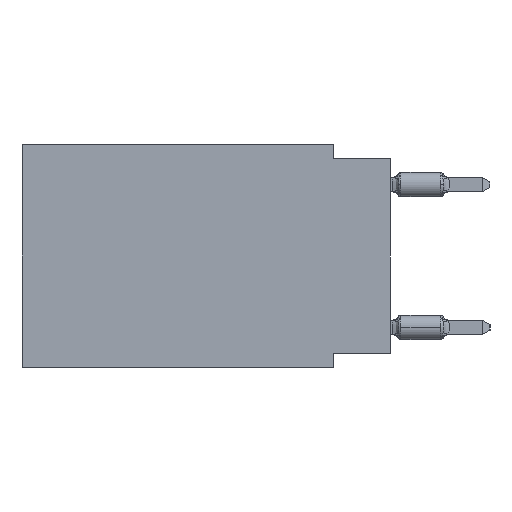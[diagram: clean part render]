
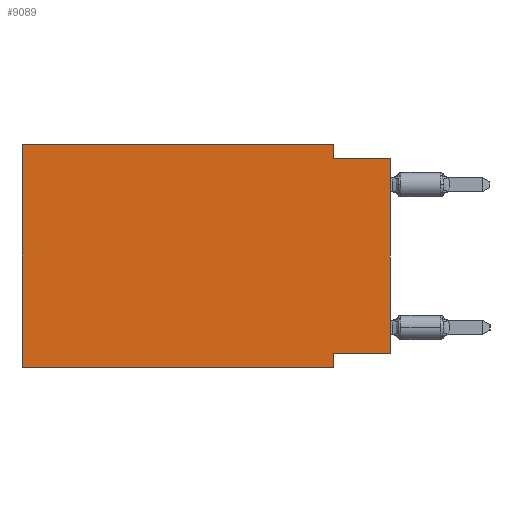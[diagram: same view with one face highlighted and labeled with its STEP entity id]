
A CAD part, left-side view. The second image highlights one B-rep face of the part: STEP entity #9089.
In plain terms, the highlighted planar face has unit normal (-1, 0, 0).
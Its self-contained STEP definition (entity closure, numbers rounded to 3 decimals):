
#278 = CARTESIAN_POINT ( 'NONE',  ( 0., 16.383, -9.906 ) ) ;
#940 = CARTESIAN_POINT ( 'NONE',  ( 0., 16.383, 0. ) ) ;
#2122 = EDGE_CURVE ( 'NONE', #52964, #34339, #27062, .T. ) ;
#2291 = DIRECTION ( 'NONE',  ( 0., 0., -1. ) ) ;
#2636 = VECTOR ( 'NONE', #54339, 1000. ) ;
#2675 = DIRECTION ( 'NONE',  ( 0., 0., -1. ) ) ;
#3881 = ORIENTED_EDGE ( 'NONE', *, *, #19318, .F. ) ;
#4041 = CARTESIAN_POINT ( 'NONE',  ( 0., 16.383, -9.906 ) ) ;
#5003 = CARTESIAN_POINT ( 'NONE',  ( 0., 0., -0.635 ) ) ;
#6231 = VERTEX_POINT ( 'NONE', #63188 ) ;
#7079 = LINE ( 'NONE', #26649, #36081 ) ;
#8442 = CARTESIAN_POINT ( 'NONE',  ( 0., 0., -9.271 ) ) ;
#8522 = ORIENTED_EDGE ( 'NONE', *, *, #10844, .F. ) ;
#9089 = ADVANCED_FACE ( 'NONE', ( #62820 ), #26673, .F. ) ;
#9523 = VERTEX_POINT ( 'NONE', #48956 ) ;
#9711 = ORIENTED_EDGE ( 'NONE', *, *, #2122, .F. ) ;
#9766 = LINE ( 'NONE', #44403, #2636 ) ;
#10844 = EDGE_CURVE ( 'NONE', #9523, #28104, #9766, .T. ) ;
#12619 = DIRECTION ( 'NONE',  ( 0., 1., 0. ) ) ;
#18020 = VERTEX_POINT ( 'NONE', #57572 ) ;
#18753 = ORIENTED_EDGE ( 'NONE', *, *, #34038, .T. ) ;
#19318 = EDGE_CURVE ( 'NONE', #6231, #9523, #47094, .T. ) ;
#19888 = ORIENTED_EDGE ( 'NONE', *, *, #21830, .F. ) ;
#20615 = CARTESIAN_POINT ( 'NONE',  ( 0., 0., 0. ) ) ;
#21154 = DIRECTION ( 'NONE',  ( 0., 0., 1. ) ) ;
#21830 = EDGE_CURVE ( 'NONE', #51669, #6231, #7079, .T. ) ;
#23291 = LINE ( 'NONE', #4041, #43035 ) ;
#25423 = LINE ( 'NONE', #20615, #36419 ) ;
#25830 = VECTOR ( 'NONE', #12619, 1000. ) ;
#26649 = CARTESIAN_POINT ( 'NONE',  ( 0., 16.383, 0. ) ) ;
#26673 = PLANE ( 'NONE',  #58840 ) ;
#27062 = LINE ( 'NONE', #56588, #57281 ) ;
#28104 = VERTEX_POINT ( 'NONE', #5003 ) ;
#28154 = CARTESIAN_POINT ( 'NONE',  ( 0., 2.54, 0. ) ) ;
#30654 = CARTESIAN_POINT ( 'NONE',  ( 0., 16.383, 0. ) ) ;
#32009 = CARTESIAN_POINT ( 'NONE',  ( 0., 2.54, -9.271 ) ) ;
#34038 = EDGE_CURVE ( 'NONE', #59448, #34339, #23291, .T. ) ;
#34339 = VERTEX_POINT ( 'NONE', #41537 ) ;
#35920 = LINE ( 'NONE', #940, #36471 ) ;
#36081 = VECTOR ( 'NONE', #56169, 1000. ) ;
#36419 = VECTOR ( 'NONE', #45328, 1000. ) ;
#36471 = VECTOR ( 'NONE', #21154, 1000. ) ;
#38458 = DIRECTION ( 'NONE',  ( 1., 0., 0. ) ) ;
#41363 = EDGE_CURVE ( 'NONE', #18020, #28104, #25423, .T. ) ;
#41537 = CARTESIAN_POINT ( 'NONE',  ( 0., 2.54, -9.906 ) ) ;
#41997 = VECTOR ( 'NONE', #61523, 1000. ) ;
#42789 = LINE ( 'NONE', #8442, #25830 ) ;
#43031 = EDGE_LOOP ( 'NONE', ( #60229, #8522, #3881, #19888, #45218, #18753, #9711, #46768 ) ) ;
#43035 = VECTOR ( 'NONE', #58577, 1000. ) ;
#44403 = CARTESIAN_POINT ( 'NONE',  ( 0., 0., -0.635 ) ) ;
#45218 = ORIENTED_EDGE ( 'NONE', *, *, #46944, .F. ) ;
#45328 = DIRECTION ( 'NONE',  ( 0., 0., 1. ) ) ;
#46768 = ORIENTED_EDGE ( 'NONE', *, *, #56820, .F. ) ;
#46944 = EDGE_CURVE ( 'NONE', #59448, #51669, #35920, .T. ) ;
#47094 = LINE ( 'NONE', #28154, #41997 ) ;
#48956 = CARTESIAN_POINT ( 'NONE',  ( 0., 2.54, -0.635 ) ) ;
#51669 = VERTEX_POINT ( 'NONE', #30654 ) ;
#52964 = VERTEX_POINT ( 'NONE', #32009 ) ;
#54339 = DIRECTION ( 'NONE',  ( 0., -1., 0. ) ) ;
#56169 = DIRECTION ( 'NONE',  ( 0., -1., 0. ) ) ;
#56588 = CARTESIAN_POINT ( 'NONE',  ( 0., 2.54, -9.906 ) ) ;
#56820 = EDGE_CURVE ( 'NONE', #18020, #52964, #42789, .T. ) ;
#57281 = VECTOR ( 'NONE', #2675, 1000. ) ;
#57572 = CARTESIAN_POINT ( 'NONE',  ( 0., 0., -9.271 ) ) ;
#58334 = CARTESIAN_POINT ( 'NONE',  ( 0., 16.383, 0. ) ) ;
#58577 = DIRECTION ( 'NONE',  ( 0., -1., 0. ) ) ;
#58840 = AXIS2_PLACEMENT_3D ( 'NONE', #58334, #38458, #2291 ) ;
#59448 = VERTEX_POINT ( 'NONE', #278 ) ;
#60229 = ORIENTED_EDGE ( 'NONE', *, *, #41363, .T. ) ;
#61523 = DIRECTION ( 'NONE',  ( 0., 0., -1. ) ) ;
#62820 = FACE_OUTER_BOUND ( 'NONE', #43031, .T. ) ;
#63188 = CARTESIAN_POINT ( 'NONE',  ( 0., 2.54, 0. ) ) ;
